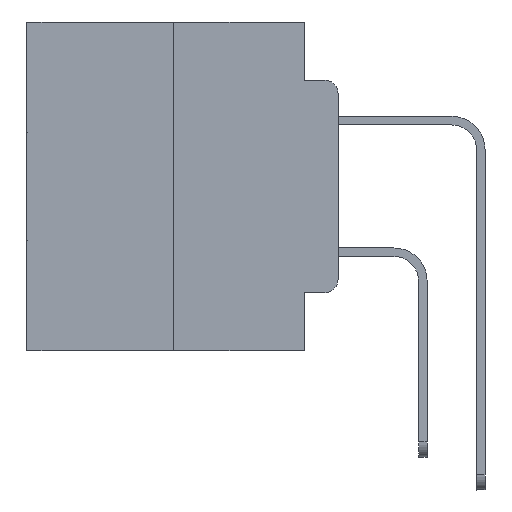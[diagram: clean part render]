
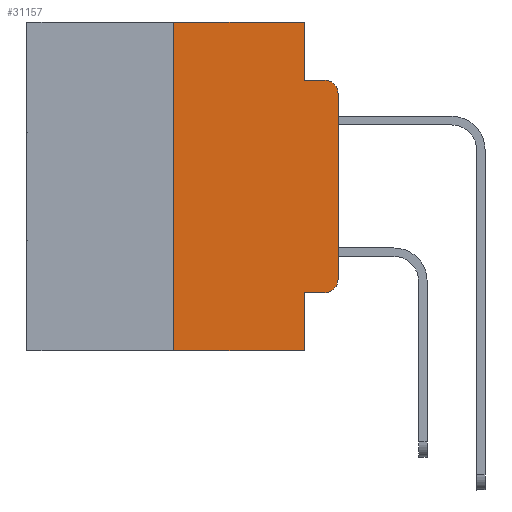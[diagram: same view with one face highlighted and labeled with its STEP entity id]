
A CAD part, left-side view. The second image highlights one B-rep face of the part: STEP entity #31157.
In plain terms, the highlighted planar face has unit normal (-1, 0, 0).
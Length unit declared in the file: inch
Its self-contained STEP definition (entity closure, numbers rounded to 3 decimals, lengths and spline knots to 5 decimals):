
#204 = ORIENTED_EDGE ( 'NONE', *, *, #11326, .T. ) ;
#368 = VERTEX_POINT ( 'NONE', #1996 ) ;
#1580 = AXIS2_PLACEMENT_3D ( 'NONE', #21846, #7297, #24250 ) ;
#1996 = CARTESIAN_POINT ( 'NONE',  ( 0., 0.051, -0.0885 ) ) ;
#2161 = CARTESIAN_POINT ( 'NONE',  ( 0., 0.051, -0.0885 ) ) ;
#2260 = VECTOR ( 'NONE', #25319, 39.37008 ) ;
#2758 = ORIENTED_EDGE ( 'NONE', *, *, #12672, .F. ) ;
#2773 = PLANE ( 'NONE',  #14375 ) ;
#2853 = VERTEX_POINT ( 'NONE', #5398 ) ;
#3130 = VECTOR ( 'NONE', #17075, 39.37008 ) ;
#3229 = CARTESIAN_POINT ( 'NONE',  ( 0., 0.02, -0.0885 ) ) ;
#3321 = LINE ( 'NONE', #3921, #14175 ) ;
#3921 = CARTESIAN_POINT ( 'NONE',  ( 0., 0.051, 0. ) ) ;
#5109 = LINE ( 'NONE', #7321, #16653 ) ;
#5315 = DIRECTION ( 'NONE',  ( 0., 0., -1. ) ) ;
#5398 = CARTESIAN_POINT ( 'NONE',  ( 0., 0.02, -0.4115 ) ) ;
#5710 = EDGE_CURVE ( 'NONE', #11746, #368, #10038, .T. ) ;
#5874 = CARTESIAN_POINT ( 'NONE',  ( 0., 0.051, -0.4115 ) ) ;
#6262 = DIRECTION ( 'NONE',  ( 0., 0., 1. ) ) ;
#6534 = CARTESIAN_POINT ( 'NONE',  ( 0., 0., -0.3915 ) ) ;
#7194 = CARTESIAN_POINT ( 'NONE',  ( 0., 0.02, -0.1085 ) ) ;
#7297 = DIRECTION ( 'NONE',  ( -1., 0., 0. ) ) ;
#7321 = CARTESIAN_POINT ( 'NONE',  ( 0., 0.473, -0.5 ) ) ;
#7662 = CARTESIAN_POINT ( 'NONE',  ( 0., 0.473, 0. ) ) ;
#8639 = DIRECTION ( 'NONE',  ( 0., 0., -1. ) ) ;
#9655 = DIRECTION ( 'NONE',  ( 0., 0., -1. ) ) ;
#9727 = CARTESIAN_POINT ( 'NONE',  ( 0., 0.473, 0. ) ) ;
#10038 = LINE ( 'NONE', #25543, #16516 ) ;
#10044 = EDGE_CURVE ( 'NONE', #368, #17347, #19851, .T. ) ;
#10099 = ORIENTED_EDGE ( 'NONE', *, *, #27303, .T. ) ;
#10670 = EDGE_CURVE ( 'NONE', #18940, #31085, #13755, .T. ) ;
#11326 = EDGE_CURVE ( 'NONE', #2853, #18940, #21254, .T. ) ;
#11404 = CARTESIAN_POINT ( 'NONE',  ( 0., 0.25, -0.5 ) ) ;
#11746 = VERTEX_POINT ( 'NONE', #25586 ) ;
#11786 = VERTEX_POINT ( 'NONE', #11404 ) ;
#11971 = VERTEX_POINT ( 'NONE', #24056 ) ;
#12154 = DIRECTION ( 'NONE',  ( 0., -1., 0. ) ) ;
#12207 = DIRECTION ( 'NONE',  ( 0., -1., 0. ) ) ;
#12557 = CARTESIAN_POINT ( 'NONE',  ( 0., 0.051, -0.4115 ) ) ;
#12672 = EDGE_CURVE ( 'NONE', #21507, #11746, #29002, .T. ) ;
#13575 = EDGE_CURVE ( 'NONE', #22898, #2853, #21866, .T. ) ;
#13733 = VECTOR ( 'NONE', #6262, 39.37008 ) ;
#13755 = LINE ( 'NONE', #31364, #25776 ) ;
#14175 = VECTOR ( 'NONE', #23483, 39.37008 ) ;
#14375 = AXIS2_PLACEMENT_3D ( 'NONE', #7662, #20000, #5315 ) ;
#14466 = AXIS2_PLACEMENT_3D ( 'NONE', #7194, #24150, #9655 ) ;
#14926 = CARTESIAN_POINT ( 'NONE',  ( 0., 0., -0.1085 ) ) ;
#15676 = ORIENTED_EDGE ( 'NONE', *, *, #18215, .F. ) ;
#16013 = CARTESIAN_POINT ( 'NONE',  ( 0., 0.25, 0. ) ) ;
#16516 = VECTOR ( 'NONE', #8639, 39.37008 ) ;
#16653 = VECTOR ( 'NONE', #12154, 39.37008 ) ;
#17006 = ORIENTED_EDGE ( 'NONE', *, *, #10670, .T. ) ;
#17075 = DIRECTION ( 'NONE',  ( 0., -1., 0. ) ) ;
#17347 = VERTEX_POINT ( 'NONE', #3229 ) ;
#18215 = EDGE_CURVE ( 'NONE', #22898, #11971, #3321, .T. ) ;
#18339 = VECTOR ( 'NONE', #12207, 39.37008 ) ;
#18940 = VERTEX_POINT ( 'NONE', #6534 ) ;
#19167 = ORIENTED_EDGE ( 'NONE', *, *, #10044, .F. ) ;
#19391 = ORIENTED_EDGE ( 'NONE', *, *, #13575, .T. ) ;
#19851 = LINE ( 'NONE', #2161, #18339 ) ;
#20000 = DIRECTION ( 'NONE',  ( 1., 0., 0. ) ) ;
#20056 = EDGE_CURVE ( 'NONE', #11786, #21507, #20173, .T. ) ;
#20173 = LINE ( 'NONE', #16013, #13733 ) ;
#20692 = CIRCLE ( 'NONE', #14466, 0.02 ) ;
#21254 = CIRCLE ( 'NONE', #1580, 0.02 ) ;
#21507 = VERTEX_POINT ( 'NONE', #23609 ) ;
#21846 = CARTESIAN_POINT ( 'NONE',  ( 0., 0.02, -0.3915 ) ) ;
#21866 = LINE ( 'NONE', #5874, #2260 ) ;
#21879 = DIRECTION ( 'NONE',  ( 0., 0., 1. ) ) ;
#22862 = ORIENTED_EDGE ( 'NONE', *, *, #25451, .T. ) ;
#22898 = VERTEX_POINT ( 'NONE', #12557 ) ;
#23417 = ORIENTED_EDGE ( 'NONE', *, *, #20056, .F. ) ;
#23483 = DIRECTION ( 'NONE',  ( 0., 0., -1. ) ) ;
#23609 = CARTESIAN_POINT ( 'NONE',  ( 0., 0.25, 0. ) ) ;
#23612 = FACE_OUTER_BOUND ( 'NONE', #28776, .T. ) ;
#24056 = CARTESIAN_POINT ( 'NONE',  ( 0., 0.051, -0.5 ) ) ;
#24150 = DIRECTION ( 'NONE',  ( -1., 0., 0. ) ) ;
#24250 = DIRECTION ( 'NONE',  ( 0., 0., -1. ) ) ;
#25319 = DIRECTION ( 'NONE',  ( 0., -1., 0. ) ) ;
#25451 = EDGE_CURVE ( 'NONE', #31085, #17347, #20692, .T. ) ;
#25543 = CARTESIAN_POINT ( 'NONE',  ( 0., 0.051, 0. ) ) ;
#25586 = CARTESIAN_POINT ( 'NONE',  ( 0., 0.051, 0. ) ) ;
#25776 = VECTOR ( 'NONE', #21879, 39.37008 ) ;
#27303 = EDGE_CURVE ( 'NONE', #11786, #11971, #5109, .T. ) ;
#27673 = ORIENTED_EDGE ( 'NONE', *, *, #5710, .F. ) ;
#28776 = EDGE_LOOP ( 'NONE', ( #17006, #22862, #19167, #27673, #2758, #23417, #10099, #15676, #19391, #204 ) ) ;
#29002 = LINE ( 'NONE', #9727, #3130 ) ;
#31085 = VERTEX_POINT ( 'NONE', #14926 ) ;
#31157 = ADVANCED_FACE ( 'NONE', ( #23612 ), #2773, .F. ) ;
#31364 = CARTESIAN_POINT ( 'NONE',  ( 0., 0., 0. ) ) ;
